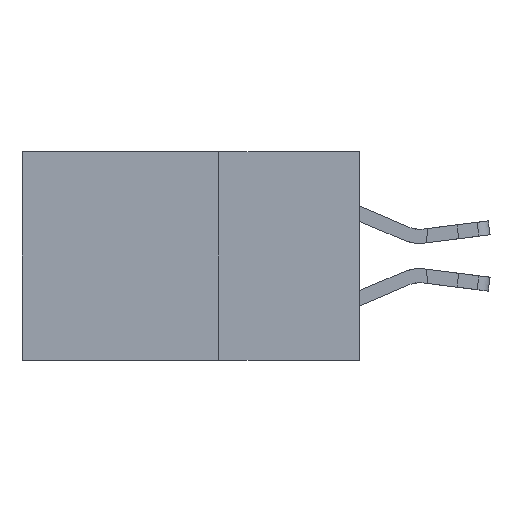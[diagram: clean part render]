
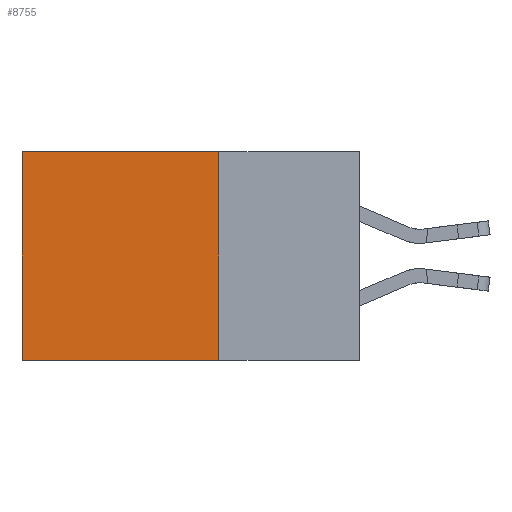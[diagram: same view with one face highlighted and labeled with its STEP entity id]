
A CAD part, left-side view. The second image highlights one B-rep face of the part: STEP entity #8755.
In plain terms, the highlighted planar face has unit normal (-1, 0, 0).
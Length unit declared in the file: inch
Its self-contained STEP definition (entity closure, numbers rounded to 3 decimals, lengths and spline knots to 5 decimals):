
#4 = VECTOR ( 'NONE', #580, 39.37008 ) ;
#580 = DIRECTION ( 'NONE',  ( 0., 0., -1. ) ) ;
#618 = ORIENTED_EDGE ( 'NONE', *, *, #17243, .T. ) ;
#1252 = CARTESIAN_POINT ( 'NONE',  ( 0.2875, 0.25, 0. ) ) ;
#1432 = ORIENTED_EDGE ( 'NONE', *, *, #11474, .F. ) ;
#2023 = CARTESIAN_POINT ( 'NONE',  ( 0.2875, 0.25, 0. ) ) ;
#2141 = CARTESIAN_POINT ( 'NONE',  ( 0.2875, 0.6, -0.37 ) ) ;
#2662 = VECTOR ( 'NONE', #12436, 39.37008 ) ;
#3532 = EDGE_CURVE ( 'NONE', #16560, #17959, #13315, .T. ) ;
#3612 = DIRECTION ( 'NONE',  ( 0., 1., 0. ) ) ;
#4076 = CARTESIAN_POINT ( 'NONE',  ( 0.2875, 0.25, -0.37 ) ) ;
#4602 = VECTOR ( 'NONE', #3612, 39.37008 ) ;
#5062 = AXIS2_PLACEMENT_3D ( 'NONE', #1252, #19278, #7384 ) ;
#6203 = LINE ( 'NONE', #4076, #14484 ) ;
#7384 = DIRECTION ( 'NONE',  ( 0., 0., -1. ) ) ;
#8670 = LINE ( 'NONE', #2023, #4602 ) ;
#8755 = ADVANCED_FACE ( 'NONE', ( #12919 ), #17898, .F. ) ;
#8882 = CARTESIAN_POINT ( 'NONE',  ( 0.2875, 0.25, 0. ) ) ;
#9093 = EDGE_LOOP ( 'NONE', ( #618, #1432, #17717, #11401 ) ) ;
#10489 = LINE ( 'NONE', #15056, #2662 ) ;
#11245 = VERTEX_POINT ( 'NONE', #15647 ) ;
#11401 = ORIENTED_EDGE ( 'NONE', *, *, #18268, .T. ) ;
#11474 = EDGE_CURVE ( 'NONE', #17959, #14798, #6203, .T. ) ;
#12436 = DIRECTION ( 'NONE',  ( 0., 0., -1. ) ) ;
#12919 = FACE_OUTER_BOUND ( 'NONE', #9093, .T. ) ;
#13006 = CARTESIAN_POINT ( 'NONE',  ( 0.2875, 0.25, 0. ) ) ;
#13116 = DIRECTION ( 'NONE',  ( 0., 1., 0. ) ) ;
#13315 = LINE ( 'NONE', #13006, #4 ) ;
#14484 = VECTOR ( 'NONE', #13116, 39.37008 ) ;
#14798 = VERTEX_POINT ( 'NONE', #2141 ) ;
#14890 = CARTESIAN_POINT ( 'NONE',  ( 0.2875, 0.25, -0.37 ) ) ;
#15056 = CARTESIAN_POINT ( 'NONE',  ( 0.2875, 0.6, 0. ) ) ;
#15647 = CARTESIAN_POINT ( 'NONE',  ( 0.2875, 0.6, 0. ) ) ;
#16560 = VERTEX_POINT ( 'NONE', #8882 ) ;
#17243 = EDGE_CURVE ( 'NONE', #11245, #14798, #10489, .T. ) ;
#17717 = ORIENTED_EDGE ( 'NONE', *, *, #3532, .F. ) ;
#17898 = PLANE ( 'NONE',  #5062 ) ;
#17959 = VERTEX_POINT ( 'NONE', #14890 ) ;
#18268 = EDGE_CURVE ( 'NONE', #16560, #11245, #8670, .T. ) ;
#19278 = DIRECTION ( 'NONE',  ( 1., 0., 0. ) ) ;
